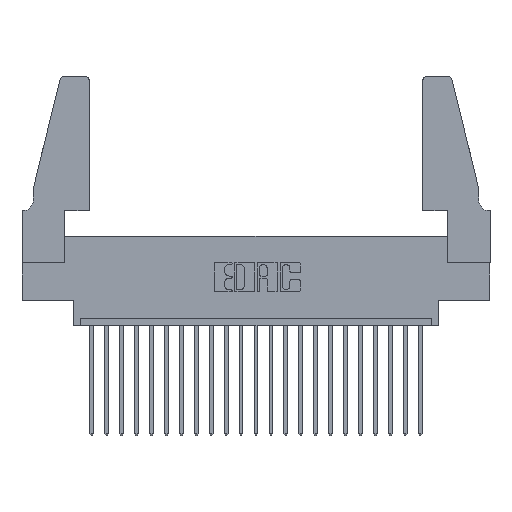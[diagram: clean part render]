
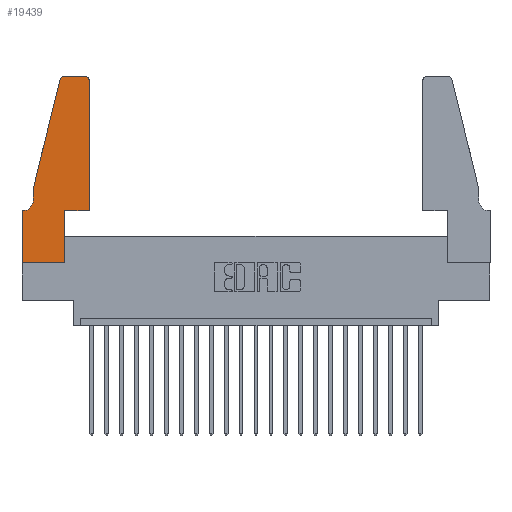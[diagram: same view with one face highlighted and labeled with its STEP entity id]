
A CAD part, top view. The second image highlights one B-rep face of the part: STEP entity #19439.
In plain terms, the highlighted planar face has unit normal (0, 0, 1).
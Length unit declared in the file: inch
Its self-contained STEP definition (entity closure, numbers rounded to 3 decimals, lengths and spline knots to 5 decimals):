
#79 = VERTEX_POINT ( 'NONE', #2216 ) ;
#272 = VERTEX_POINT ( 'NONE', #21580 ) ;
#416 = CARTESIAN_POINT ( 'NONE',  ( 0.0755, 0.35, 0.37 ) ) ;
#820 = EDGE_CURVE ( 'NONE', #272, #14248, #3874, .T. ) ;
#920 = EDGE_CURVE ( 'NONE', #16742, #79, #8174, .T. ) ;
#1946 = EDGE_CURVE ( 'NONE', #8806, #5213, #21477, .T. ) ;
#2154 = ORIENTED_EDGE ( 'NONE', *, *, #4445, .T. ) ;
#2163 = LINE ( 'NONE', #416, #16960 ) ;
#2216 = CARTESIAN_POINT ( 'NONE',  ( 0.4205, 1.25, 0.37 ) ) ;
#2219 = AXIS2_PLACEMENT_3D ( 'NONE', #14515, #21492, #12973 ) ;
#2421 = CARTESIAN_POINT ( 'NONE',  ( 0.284, 1.22, 0.37 ) ) ;
#3155 = CARTESIAN_POINT ( 'NONE',  ( 0.284, 1.25, 0.37 ) ) ;
#3309 = DIRECTION ( 'NONE',  ( -0.239, -0.971, 0. ) ) ;
#3874 = CIRCLE ( 'NONE', #2219, 0.07 ) ;
#3901 = CARTESIAN_POINT ( 'NONE',  ( 0., 0., 0.37 ) ) ;
#4252 = VECTOR ( 'NONE', #12871, 39.37008 ) ;
#4266 = LINE ( 'NONE', #10757, #14450 ) ;
#4445 = EDGE_CURVE ( 'NONE', #5213, #4735, #9584, .T. ) ;
#4529 = VERTEX_POINT ( 'NONE', #3901 ) ;
#4735 = VERTEX_POINT ( 'NONE', #14405 ) ;
#4751 = AXIS2_PLACEMENT_3D ( 'NONE', #20302, #6646, #18399 ) ;
#4971 = CARTESIAN_POINT ( 'NONE',  ( 0., 0., 0.37 ) ) ;
#5213 = VERTEX_POINT ( 'NONE', #11235 ) ;
#5607 = ORIENTED_EDGE ( 'NONE', *, *, #10986, .T. ) ;
#5752 = VECTOR ( 'NONE', #19596, 39.37008 ) ;
#5994 = ORIENTED_EDGE ( 'NONE', *, *, #19647, .T. ) ;
#6234 = EDGE_CURVE ( 'NONE', #9956, #8223, #7172, .T. ) ;
#6560 = CARTESIAN_POINT ( 'NONE',  ( 0.2865, 0.35, 0.37 ) ) ;
#6575 = PLANE ( 'NONE',  #4751 ) ;
#6591 = CARTESIAN_POINT ( 'NONE',  ( 0.4505, 0.35, 0.37 ) ) ;
#6646 = DIRECTION ( 'NONE',  ( 0., 0., 1. ) ) ;
#6890 = CARTESIAN_POINT ( 'NONE',  ( 0.2865, 0.35, 0.37 ) ) ;
#7006 = VECTOR ( 'NONE', #19077, 39.37008 ) ;
#7172 = LINE ( 'NONE', #12810, #16853 ) ;
#7874 = ORIENTED_EDGE ( 'NONE', *, *, #1946, .T. ) ;
#7990 = CARTESIAN_POINT ( 'NONE',  ( 0.4205, 1.22, 0.37 ) ) ;
#8003 = AXIS2_PLACEMENT_3D ( 'NONE', #7990, #11591, #16559 ) ;
#8174 = CIRCLE ( 'NONE', #8003, 0.03 ) ;
#8223 = VERTEX_POINT ( 'NONE', #9426 ) ;
#8356 = ORIENTED_EDGE ( 'NONE', *, *, #20506, .T. ) ;
#8806 = VERTEX_POINT ( 'NONE', #3155 ) ;
#8965 = DIRECTION ( 'NONE',  ( 0., -1., 0. ) ) ;
#9185 = DIRECTION ( 'NONE',  ( 0., -1., 0. ) ) ;
#9389 = CARTESIAN_POINT ( 'NONE',  ( 0., 0.35, 0.37 ) ) ;
#9426 = CARTESIAN_POINT ( 'NONE',  ( 0.4505, 0.35, 0.37 ) ) ;
#9584 = LINE ( 'NONE', #13486, #15254 ) ;
#9956 = VERTEX_POINT ( 'NONE', #6560 ) ;
#10214 = EDGE_CURVE ( 'NONE', #14248, #10545, #2163, .T. ) ;
#10293 = ORIENTED_EDGE ( 'NONE', *, *, #10404, .T. ) ;
#10404 = EDGE_CURVE ( 'NONE', #18780, #9956, #20131, .T. ) ;
#10545 = VERTEX_POINT ( 'NONE', #9389 ) ;
#10757 = CARTESIAN_POINT ( 'NONE',  ( 0.0755, 0.5, 0.37 ) ) ;
#10986 = EDGE_CURVE ( 'NONE', #4735, #272, #4266, .T. ) ;
#11235 = CARTESIAN_POINT ( 'NONE',  ( 0.25487, 1.22718, 0.37 ) ) ;
#11361 = FACE_OUTER_BOUND ( 'NONE', #19372, .T. ) ;
#11575 = LINE ( 'NONE', #12614, #5752 ) ;
#11591 = DIRECTION ( 'NONE',  ( 0., 0., 1. ) ) ;
#12614 = CARTESIAN_POINT ( 'NONE',  ( 0.2605, 1.25, 0.37 ) ) ;
#12810 = CARTESIAN_POINT ( 'NONE',  ( 0.4505, 0.35, 0.37 ) ) ;
#12871 = DIRECTION ( 'NONE',  ( 1., 0., 0. ) ) ;
#12973 = DIRECTION ( 'NONE',  ( -1., 0., 0. ) ) ;
#13268 = VECTOR ( 'NONE', #8965, 39.37008 ) ;
#13289 = ORIENTED_EDGE ( 'NONE', *, *, #820, .T. ) ;
#13333 = ORIENTED_EDGE ( 'NONE', *, *, #14031, .T. ) ;
#13486 = CARTESIAN_POINT ( 'NONE',  ( 0.0755, 0.5, 0.37 ) ) ;
#13493 = AXIS2_PLACEMENT_3D ( 'NONE', #2421, #17887, #19573 ) ;
#13567 = ORIENTED_EDGE ( 'NONE', *, *, #6234, .T. ) ;
#14031 = EDGE_CURVE ( 'NONE', #8223, #16742, #17988, .T. ) ;
#14248 = VERTEX_POINT ( 'NONE', #17425 ) ;
#14405 = CARTESIAN_POINT ( 'NONE',  ( 0.0755, 0.5, 0.37 ) ) ;
#14409 = CARTESIAN_POINT ( 'NONE',  ( 0.4505, 1.22, 0.37 ) ) ;
#14450 = VECTOR ( 'NONE', #9185, 39.37008 ) ;
#14515 = CARTESIAN_POINT ( 'NONE',  ( 0.0055, 0.42, 0.37 ) ) ;
#14942 = CARTESIAN_POINT ( 'NONE',  ( 0.2865, 0., 0.37 ) ) ;
#15068 = EDGE_CURVE ( 'NONE', #4529, #18780, #19243, .T. ) ;
#15253 = ORIENTED_EDGE ( 'NONE', *, *, #15068, .T. ) ;
#15254 = VECTOR ( 'NONE', #3309, 39.37008 ) ;
#15823 = DIRECTION ( 'NONE',  ( -1., 0., 0. ) ) ;
#16498 = ORIENTED_EDGE ( 'NONE', *, *, #920, .T. ) ;
#16559 = DIRECTION ( 'NONE',  ( 1., 0., 0. ) ) ;
#16690 = ORIENTED_EDGE ( 'NONE', *, *, #10214, .T. ) ;
#16742 = VERTEX_POINT ( 'NONE', #14409 ) ;
#16853 = VECTOR ( 'NONE', #17799, 39.37008 ) ;
#16960 = VECTOR ( 'NONE', #15823, 39.37008 ) ;
#17425 = CARTESIAN_POINT ( 'NONE',  ( 0.0055, 0.35, 0.37 ) ) ;
#17799 = DIRECTION ( 'NONE',  ( 1., 0., 0. ) ) ;
#17857 = LINE ( 'NONE', #4971, #13268 ) ;
#17887 = DIRECTION ( 'NONE',  ( 0., 0., 1. ) ) ;
#17988 = LINE ( 'NONE', #6591, #20097 ) ;
#18399 = DIRECTION ( 'NONE',  ( 1., 0., 0. ) ) ;
#18780 = VERTEX_POINT ( 'NONE', #14942 ) ;
#19077 = DIRECTION ( 'NONE',  ( 0., 1., 0. ) ) ;
#19243 = LINE ( 'NONE', #21542, #4252 ) ;
#19372 = EDGE_LOOP ( 'NONE', ( #8356, #7874, #2154, #5607, #13289, #16690, #5994, #15253, #10293, #13567, #13333, #16498 ) ) ;
#19439 = ADVANCED_FACE ( 'NONE', ( #11361 ), #6575, .T. ) ;
#19573 = DIRECTION ( 'NONE',  ( 1., 0., 0. ) ) ;
#19596 = DIRECTION ( 'NONE',  ( -1., 0., 0. ) ) ;
#19647 = EDGE_CURVE ( 'NONE', #10545, #4529, #17857, .T. ) ;
#20097 = VECTOR ( 'NONE', #21584, 39.37008 ) ;
#20131 = LINE ( 'NONE', #6890, #7006 ) ;
#20302 = CARTESIAN_POINT ( 'NONE',  ( 0., 0.35, 0.37 ) ) ;
#20506 = EDGE_CURVE ( 'NONE', #79, #8806, #11575, .T. ) ;
#21477 = CIRCLE ( 'NONE', #13493, 0.03 ) ;
#21492 = DIRECTION ( 'NONE',  ( 0., 0., -1. ) ) ;
#21542 = CARTESIAN_POINT ( 'NONE',  ( 0., 0., 0.37 ) ) ;
#21580 = CARTESIAN_POINT ( 'NONE',  ( 0.0755, 0.42, 0.37 ) ) ;
#21584 = DIRECTION ( 'NONE',  ( 0., 1., 0. ) ) ;
